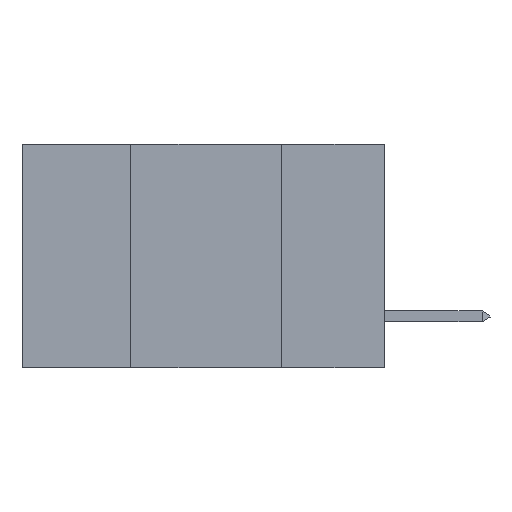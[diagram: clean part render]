
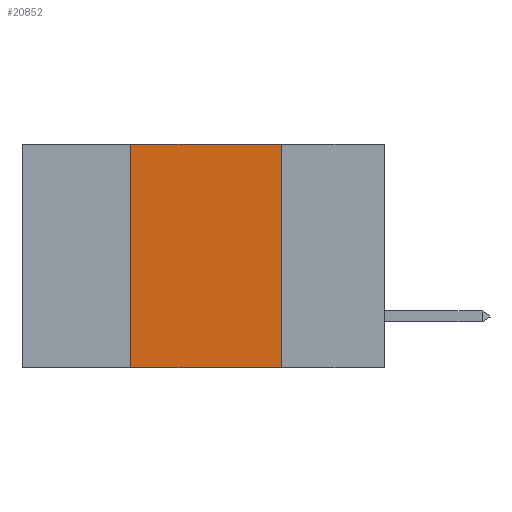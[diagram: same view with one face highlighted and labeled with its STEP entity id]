
A CAD part, left-side view. The second image highlights one B-rep face of the part: STEP entity #20852.
In plain terms, the highlighted planar face has unit normal (-1, 0, 0).
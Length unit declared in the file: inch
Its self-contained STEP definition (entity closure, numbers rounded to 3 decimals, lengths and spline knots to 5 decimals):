
#183 = CARTESIAN_POINT ( 'NONE',  ( 0., 0.6, 0. ) ) ;
#2209 = ORIENTED_EDGE ( 'NONE', *, *, #17162, .T. ) ;
#5902 = EDGE_CURVE ( 'NONE', #9383, #26492, #31105, .T. ) ;
#6621 = VECTOR ( 'NONE', #14839, 39.37008 ) ;
#6720 = VECTOR ( 'NONE', #15773, 39.37008 ) ;
#8451 = CARTESIAN_POINT ( 'NONE',  ( 0., 0.6, -0.37 ) ) ;
#9046 = CARTESIAN_POINT ( 'NONE',  ( 0., 0.42, -0.37 ) ) ;
#9383 = VERTEX_POINT ( 'NONE', #9046 ) ;
#10600 = ORIENTED_EDGE ( 'NONE', *, *, #30694, .F. ) ;
#11405 = DIRECTION ( 'NONE',  ( 1., 0., 0. ) ) ;
#11531 = AXIS2_PLACEMENT_3D ( 'NONE', #16056, #11405, #26353 ) ;
#13096 = DIRECTION ( 'NONE',  ( 0., 0., -1. ) ) ;
#13586 = PLANE ( 'NONE',  #11531 ) ;
#14839 = DIRECTION ( 'NONE',  ( 0., -1., 0. ) ) ;
#15341 = EDGE_CURVE ( 'NONE', #17403, #30230, #27994, .T. ) ;
#15773 = DIRECTION ( 'NONE',  ( 0., -1., 0. ) ) ;
#15933 = FACE_OUTER_BOUND ( 'NONE', #19735, .T. ) ;
#16056 = CARTESIAN_POINT ( 'NONE',  ( 0., 0.6, 0. ) ) ;
#16887 = CARTESIAN_POINT ( 'NONE',  ( 0., 0.17, 0. ) ) ;
#17036 = DIRECTION ( 'NONE',  ( 0., 0., 1. ) ) ;
#17162 = EDGE_CURVE ( 'NONE', #9383, #30230, #18653, .T. ) ;
#17228 = ORIENTED_EDGE ( 'NONE', *, *, #5902, .F. ) ;
#17403 = VERTEX_POINT ( 'NONE', #16887 ) ;
#18653 = LINE ( 'NONE', #8451, #6720 ) ;
#19664 = CARTESIAN_POINT ( 'NONE',  ( 0., 0.42, 0. ) ) ;
#19735 = EDGE_LOOP ( 'NONE', ( #29158, #10600, #17228, #2209 ) ) ;
#20852 = ADVANCED_FACE ( 'NONE', ( #15933 ), #13586, .F. ) ;
#22060 = CARTESIAN_POINT ( 'NONE',  ( 0., 0.17, -0.37 ) ) ;
#24575 = VECTOR ( 'NONE', #17036, 39.37008 ) ;
#25451 = LINE ( 'NONE', #183, #6621 ) ;
#26353 = DIRECTION ( 'NONE',  ( 0., 0., -1. ) ) ;
#26492 = VERTEX_POINT ( 'NONE', #19664 ) ;
#27002 = CARTESIAN_POINT ( 'NONE',  ( 0., 0.42, 0. ) ) ;
#27236 = VECTOR ( 'NONE', #13096, 39.37008 ) ;
#27994 = LINE ( 'NONE', #29943, #27236 ) ;
#29158 = ORIENTED_EDGE ( 'NONE', *, *, #15341, .F. ) ;
#29943 = CARTESIAN_POINT ( 'NONE',  ( 0., 0.17, 0. ) ) ;
#30230 = VERTEX_POINT ( 'NONE', #22060 ) ;
#30694 = EDGE_CURVE ( 'NONE', #26492, #17403, #25451, .T. ) ;
#31105 = LINE ( 'NONE', #27002, #24575 ) ;
